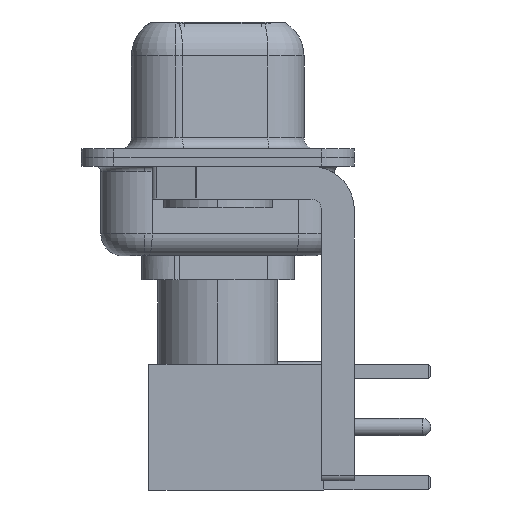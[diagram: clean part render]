
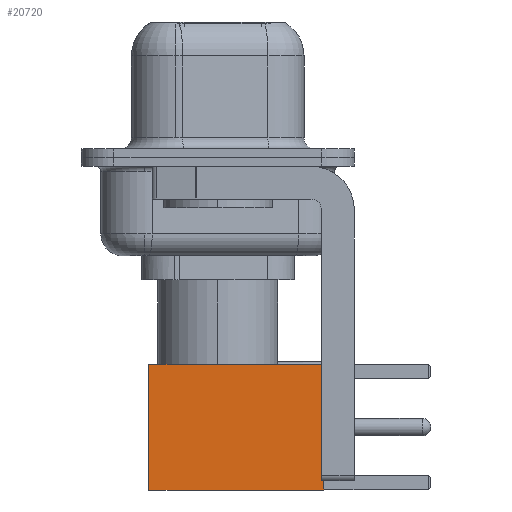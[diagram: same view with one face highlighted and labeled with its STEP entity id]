
A CAD part, left-side view. The second image highlights one B-rep face of the part: STEP entity #20720.
In plain terms, the highlighted face is planar.
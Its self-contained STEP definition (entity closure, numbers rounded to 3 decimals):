
#576 = VECTOR ( 'NONE', #11971, 1000. ) ;
#1009 = DIRECTION ( 'NONE',  ( 0., 1., 0. ) ) ;
#1225 = PLANE ( 'NONE',  #19070 ) ;
#1411 = LINE ( 'NONE', #3400, #20628 ) ;
#2543 = ORIENTED_EDGE ( 'NONE', *, *, #12225, .T. ) ;
#3181 = DIRECTION ( 'NONE',  ( -1., 0., 0. ) ) ;
#3400 = CARTESIAN_POINT ( 'NONE',  ( 0., 2.875, 8. ) ) ;
#3857 = ORIENTED_EDGE ( 'NONE', *, *, #9936, .T. ) ;
#4093 = VECTOR ( 'NONE', #4890, 1000. ) ;
#4795 = EDGE_CURVE ( 'NONE', #20700, #15860, #1411, .T. ) ;
#4890 = DIRECTION ( 'NONE',  ( -1., 0., 0. ) ) ;
#5004 = CARTESIAN_POINT ( 'NONE',  ( 0., 2.875, 0. ) ) ;
#5177 = CARTESIAN_POINT ( 'NONE',  ( 2.875, 2.875, 0. ) ) ;
#5902 = FACE_OUTER_BOUND ( 'NONE', #21696, .T. ) ;
#6987 = CARTESIAN_POINT ( 'NONE',  ( -2.875, 2.875, 0. ) ) ;
#8122 = VERTEX_POINT ( 'NONE', #6987 ) ;
#9770 = LINE ( 'NONE', #16569, #17963 ) ;
#9936 = EDGE_CURVE ( 'NONE', #21074, #8122, #9996, .T. ) ;
#9996 = LINE ( 'NONE', #5004, #4093 ) ;
#10749 = CARTESIAN_POINT ( 'NONE',  ( -2.875, 2.875, 8. ) ) ;
#11131 = CARTESIAN_POINT ( 'NONE',  ( 2.875, 2.875, 0. ) ) ;
#11853 = LINE ( 'NONE', #5177, #576 ) ;
#11971 = DIRECTION ( 'NONE',  ( 0., 0., -1. ) ) ;
#12225 = EDGE_CURVE ( 'NONE', #20700, #21074, #11853, .T. ) ;
#13135 = CARTESIAN_POINT ( 'NONE',  ( 2.875, 2.875, 8. ) ) ;
#14592 = DIRECTION ( 'NONE',  ( 0., 0., 1. ) ) ;
#14824 = ORIENTED_EDGE ( 'NONE', *, *, #4795, .F. ) ;
#15379 = ORIENTED_EDGE ( 'NONE', *, *, #19510, .F. ) ;
#15860 = VERTEX_POINT ( 'NONE', #10749 ) ;
#16569 = CARTESIAN_POINT ( 'NONE',  ( -2.875, 2.875, 0. ) ) ;
#17963 = VECTOR ( 'NONE', #21687, 1000. ) ;
#19070 = AXIS2_PLACEMENT_3D ( 'NONE', #11131, #1009, #14592 ) ;
#19510 = EDGE_CURVE ( 'NONE', #15860, #8122, #9770, .T. ) ;
#20628 = VECTOR ( 'NONE', #3181, 1000. ) ;
#20700 = VERTEX_POINT ( 'NONE', #13135 ) ;
#20720 = ADVANCED_FACE ( 'NONE', ( #5902 ), #1225, .T. ) ;
#21016 = CARTESIAN_POINT ( 'NONE',  ( 2.875, 2.875, 0. ) ) ;
#21074 = VERTEX_POINT ( 'NONE', #21016 ) ;
#21687 = DIRECTION ( 'NONE',  ( 0., 0., -1. ) ) ;
#21696 = EDGE_LOOP ( 'NONE', ( #2543, #3857, #15379, #14824 ) ) ;
